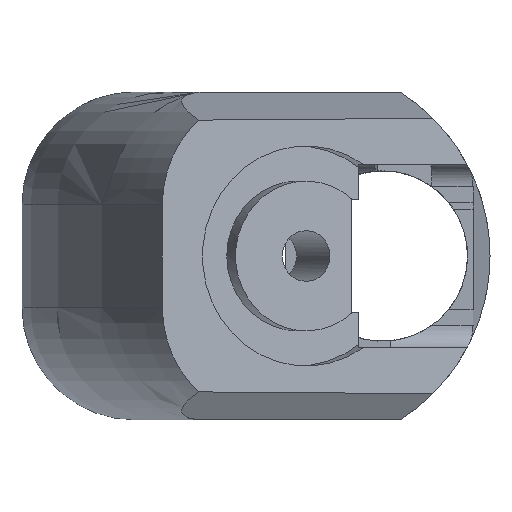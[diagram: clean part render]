
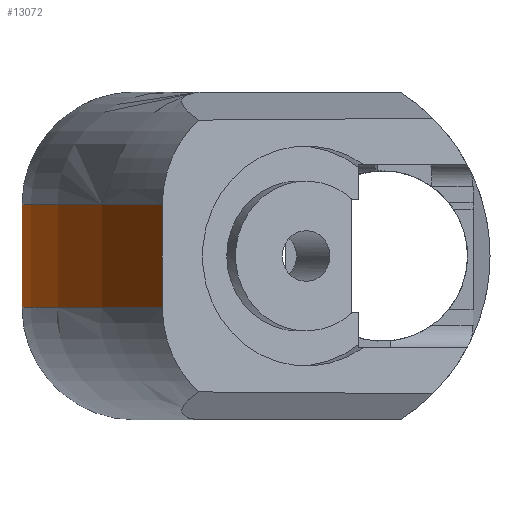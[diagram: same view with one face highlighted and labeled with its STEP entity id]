
A CAD part, left-side view. The second image highlights one B-rep face of the part: STEP entity #13072.
In plain terms, the highlighted cylindrical face has radius 197.297 mm (diameter 394.594 mm), a partial arc.
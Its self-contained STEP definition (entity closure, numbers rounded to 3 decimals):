
#157 = TOROIDAL_SURFACE('',#158,182.057,15.24);
#158 = AXIS2_PLACEMENT_3D('',#159,#160,#161);
#159 = CARTESIAN_POINT('',(-124.968,-133.797,-6.985));
#160 = DIRECTION('',(0.,0.,1.));
#161 = DIRECTION('',(0.,1.,0.));
#1723 = PLANE('',#1724);
#1724 = AXIS2_PLACEMENT_3D('',#1725,#1726,#1727);
#1725 = CARTESIAN_POINT('',(-209.55,44.45,-22.225));
#1726 = DIRECTION('',(0.943,0.334,0.)
  );
#1727 = DIRECTION('',(0.334,-0.943,0.)
  );
#2047 = PLANE('',#2048);
#2048 = AXIS2_PLACEMENT_3D('',#2049,#2050,#2051);
#2049 = CARTESIAN_POINT('',(0.,63.5,-22.225));
#2050 = DIRECTION('',(0.,-1.,0.));
#2051 = DIRECTION('',(-1.,0.,0.));
#3686 = VERTEX_POINT('',#3687);
#3687 = CARTESIAN_POINT('',(-124.968,63.5,-6.985));
#3735 = VERTEX_POINT('',#3736);
#3736 = CARTESIAN_POINT('',(-209.55,44.45,-6.985));
#3894 = EDGE_CURVE('',#3686,#3735,#3895,.T.);
#3895 = SURFACE_CURVE('',#3896,(#3901,#3908),.PCURVE_S1.);
#3896 = CIRCLE('',#3897,197.297);
#3897 = AXIS2_PLACEMENT_3D('',#3898,#3899,#3900);
#3898 = CARTESIAN_POINT('',(-124.968,-133.797,-6.985));
#3899 = DIRECTION('',(0.,0.,1.));
#3900 = DIRECTION('',(0.,1.,0.));
#3901 = PCURVE('',#157,#3902);
#3902 = DEFINITIONAL_REPRESENTATION('',(#3903),#3907);
#3903 = LINE('',#3904,#3905);
#3904 = CARTESIAN_POINT('',(0.,6.283));
#3905 = VECTOR('',#3906,1.);
#3906 = DIRECTION('',(1.,0.));
#3907 = ( GEOMETRIC_REPRESENTATION_CONTEXT(2) 
PARAMETRIC_REPRESENTATION_CONTEXT() REPRESENTATION_CONTEXT('2D SPACE',''
  ) );
#3908 = PCURVE('',#3909,#3914);
#3909 = CYLINDRICAL_SURFACE('',#3910,197.297);
#3910 = AXIS2_PLACEMENT_3D('',#3911,#3912,#3913);
#3911 = CARTESIAN_POINT('',(-124.968,-133.797,-22.225));
#3912 = DIRECTION('',(0.,0.,-1.));
#3913 = DIRECTION('',(1.,0.,0.));
#3914 = DEFINITIONAL_REPRESENTATION('',(#3915),#3919);
#3915 = LINE('',#3916,#3917);
#3916 = CARTESIAN_POINT('',(-1.571,-15.24));
#3917 = VECTOR('',#3918,1.);
#3918 = DIRECTION('',(-1.,0.));
#3919 = ( GEOMETRIC_REPRESENTATION_CONTEXT(2) 
PARAMETRIC_REPRESENTATION_CONTEXT() REPRESENTATION_CONTEXT('2D SPACE',''
  ) );
#4642 = EDGE_CURVE('',#3735,#4643,#4645,.T.);
#4643 = VERTEX_POINT('',#4644);
#4644 = CARTESIAN_POINT('',(-209.55,44.45,6.985));
#4645 = SURFACE_CURVE('',#4646,(#4650,#4657),.PCURVE_S1.);
#4646 = LINE('',#4647,#4648);
#4647 = CARTESIAN_POINT('',(-209.55,44.45,-22.225));
#4648 = VECTOR('',#4649,1.);
#4649 = DIRECTION('',(0.,0.,1.));
#4650 = PCURVE('',#1723,#4651);
#4651 = DEFINITIONAL_REPRESENTATION('',(#4652),#4656);
#4652 = LINE('',#4653,#4654);
#4653 = CARTESIAN_POINT('',(0.,-0.));
#4654 = VECTOR('',#4655,1.);
#4655 = DIRECTION('',(0.,-1.));
#4656 = ( GEOMETRIC_REPRESENTATION_CONTEXT(2) 
PARAMETRIC_REPRESENTATION_CONTEXT() REPRESENTATION_CONTEXT('2D SPACE',''
  ) );
#4657 = PCURVE('',#3909,#4658);
#4658 = DEFINITIONAL_REPRESENTATION('',(#4659),#4663);
#4659 = LINE('',#4660,#4661);
#4660 = CARTESIAN_POINT('',(-2.014,0.));
#4661 = VECTOR('',#4662,1.);
#4662 = DIRECTION('',(-0.,-1.));
#4663 = ( GEOMETRIC_REPRESENTATION_CONTEXT(2) 
PARAMETRIC_REPRESENTATION_CONTEXT() REPRESENTATION_CONTEXT('2D SPACE',''
  ) );
#4719 = TOROIDAL_SURFACE('',#4720,182.057,15.24);
#4720 = AXIS2_PLACEMENT_3D('',#4721,#4722,#4723);
#4721 = CARTESIAN_POINT('',(-124.968,-133.797,6.985));
#4722 = DIRECTION('',(0.,0.,-1.));
#4723 = DIRECTION('',(0.,1.,0.));
#6721 = VERTEX_POINT('',#6722);
#6722 = CARTESIAN_POINT('',(-124.968,63.5,6.985));
#6743 = EDGE_CURVE('',#3686,#6721,#6744,.T.);
#6744 = SURFACE_CURVE('',#6745,(#6749,#6756),.PCURVE_S1.);
#6745 = LINE('',#6746,#6747);
#6746 = CARTESIAN_POINT('',(-124.968,63.5,-22.225));
#6747 = VECTOR('',#6748,1.);
#6748 = DIRECTION('',(0.,0.,1.));
#6749 = PCURVE('',#2047,#6750);
#6750 = DEFINITIONAL_REPRESENTATION('',(#6751),#6755);
#6751 = LINE('',#6752,#6753);
#6752 = CARTESIAN_POINT('',(124.968,0.));
#6753 = VECTOR('',#6754,1.);
#6754 = DIRECTION('',(0.,-1.));
#6755 = ( GEOMETRIC_REPRESENTATION_CONTEXT(2) 
PARAMETRIC_REPRESENTATION_CONTEXT() REPRESENTATION_CONTEXT('2D SPACE',''
  ) );
#6756 = PCURVE('',#3909,#6757);
#6757 = DEFINITIONAL_REPRESENTATION('',(#6758),#6762);
#6758 = LINE('',#6759,#6760);
#6759 = CARTESIAN_POINT('',(-1.571,0.));
#6760 = VECTOR('',#6761,1.);
#6761 = DIRECTION('',(-0.,-1.));
#6762 = ( GEOMETRIC_REPRESENTATION_CONTEXT(2) 
PARAMETRIC_REPRESENTATION_CONTEXT() REPRESENTATION_CONTEXT('2D SPACE',''
  ) );
#13072 = ADVANCED_FACE('',(#13073),#3909,.T.);
#13073 = FACE_BOUND('',#13074,.F.);
#13074 = EDGE_LOOP('',(#13075,#13076,#13098,#13099));
#13075 = ORIENTED_EDGE('',*,*,#6743,.T.);
#13076 = ORIENTED_EDGE('',*,*,#13077,.T.);
#13077 = EDGE_CURVE('',#6721,#4643,#13078,.T.);
#13078 = SURFACE_CURVE('',#13079,(#13084,#13091),.PCURVE_S1.);
#13079 = CIRCLE('',#13080,197.297);
#13080 = AXIS2_PLACEMENT_3D('',#13081,#13082,#13083);
#13081 = CARTESIAN_POINT('',(-124.968,-133.797,6.985));
#13082 = DIRECTION('',(0.,0.,1.));
#13083 = DIRECTION('',(0.,1.,0.));
#13084 = PCURVE('',#3909,#13085);
#13085 = DEFINITIONAL_REPRESENTATION('',(#13086),#13090);
#13086 = LINE('',#13087,#13088);
#13087 = CARTESIAN_POINT('',(-1.571,-29.21));
#13088 = VECTOR('',#13089,1.);
#13089 = DIRECTION('',(-1.,0.));
#13090 = ( GEOMETRIC_REPRESENTATION_CONTEXT(2) 
PARAMETRIC_REPRESENTATION_CONTEXT() REPRESENTATION_CONTEXT('2D SPACE',''
  ) );
#13091 = PCURVE('',#4719,#13092);
#13092 = DEFINITIONAL_REPRESENTATION('',(#13093),#13097);
#13093 = LINE('',#13094,#13095);
#13094 = CARTESIAN_POINT('',(-0.,6.283));
#13095 = VECTOR('',#13096,1.);
#13096 = DIRECTION('',(-1.,0.));
#13097 = ( GEOMETRIC_REPRESENTATION_CONTEXT(2) 
PARAMETRIC_REPRESENTATION_CONTEXT() REPRESENTATION_CONTEXT('2D SPACE',''
  ) );
#13098 = ORIENTED_EDGE('',*,*,#4642,.F.);
#13099 = ORIENTED_EDGE('',*,*,#3894,.F.);
